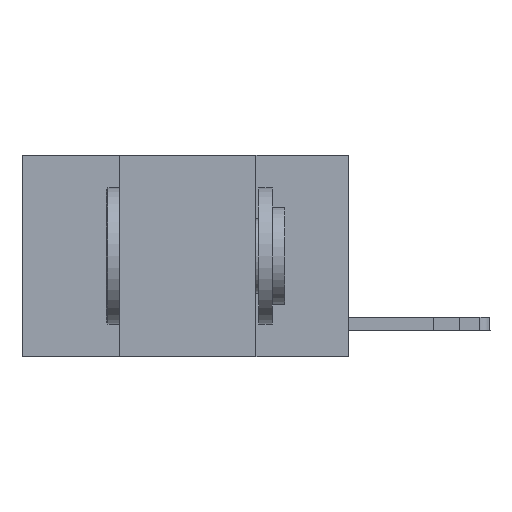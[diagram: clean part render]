
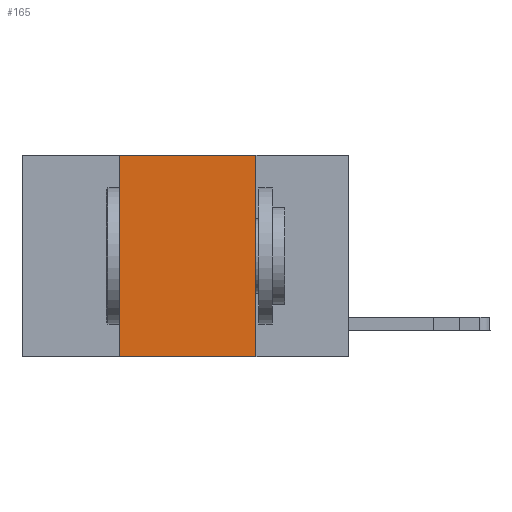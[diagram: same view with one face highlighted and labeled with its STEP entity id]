
A CAD part, left-side view. The second image highlights one B-rep face of the part: STEP entity #165.
In plain terms, the highlighted planar face has unit normal (-1, 0, 0).
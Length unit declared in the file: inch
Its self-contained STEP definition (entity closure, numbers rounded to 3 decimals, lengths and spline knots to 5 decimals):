
#32 = LINE ( 'NONE', #14705, #11902 ) ;
#165 = ADVANCED_FACE ( 'NONE', ( #14296 ), #7506, .F. ) ;
#286 = DIRECTION ( 'NONE',  ( 0., 0., -1. ) ) ;
#1054 = VERTEX_POINT ( 'NONE', #12164 ) ;
#1081 = DIRECTION ( 'NONE',  ( 0., 0., -1. ) ) ;
#1426 = CARTESIAN_POINT ( 'NONE',  ( 0., 0.17, 0. ) ) ;
#1650 = DIRECTION ( 'NONE',  ( 0., 0., 1. ) ) ;
#1777 = EDGE_LOOP ( 'NONE', ( #5308, #9752, #3244, #13307 ) ) ;
#1889 = LINE ( 'NONE', #4613, #5074 ) ;
#1970 = EDGE_CURVE ( 'NONE', #2751, #3465, #32, .T. ) ;
#2751 = VERTEX_POINT ( 'NONE', #1426 ) ;
#3244 = ORIENTED_EDGE ( 'NONE', *, *, #13881, .F. ) ;
#3465 = VERTEX_POINT ( 'NONE', #9005 ) ;
#3810 = CARTESIAN_POINT ( 'NONE',  ( 0., 0.6, 0. ) ) ;
#4613 = CARTESIAN_POINT ( 'NONE',  ( 0., 0.6, -0.37 ) ) ;
#4658 = VECTOR ( 'NONE', #1650, 39.37008 ) ;
#4887 = VECTOR ( 'NONE', #6370, 39.37008 ) ;
#4927 = CARTESIAN_POINT ( 'NONE',  ( 0., 0.6, 0. ) ) ;
#5074 = VECTOR ( 'NONE', #6948, 39.37008 ) ;
#5227 = VERTEX_POINT ( 'NONE', #6787 ) ;
#5308 = ORIENTED_EDGE ( 'NONE', *, *, #1970, .F. ) ;
#6046 = DIRECTION ( 'NONE',  ( 1., 0., 0. ) ) ;
#6195 = LINE ( 'NONE', #3810, #4887 ) ;
#6370 = DIRECTION ( 'NONE',  ( 0., -1., 0. ) ) ;
#6787 = CARTESIAN_POINT ( 'NONE',  ( 0., 0.42, -0.37 ) ) ;
#6948 = DIRECTION ( 'NONE',  ( 0., -1., 0. ) ) ;
#7162 = EDGE_CURVE ( 'NONE', #5227, #3465, #1889, .T. ) ;
#7506 = PLANE ( 'NONE',  #15822 ) ;
#9005 = CARTESIAN_POINT ( 'NONE',  ( 0., 0.17, -0.37 ) ) ;
#9684 = LINE ( 'NONE', #10653, #4658 ) ;
#9752 = ORIENTED_EDGE ( 'NONE', *, *, #10491, .F. ) ;
#10491 = EDGE_CURVE ( 'NONE', #1054, #2751, #6195, .T. ) ;
#10653 = CARTESIAN_POINT ( 'NONE',  ( 0., 0.42, 0. ) ) ;
#11902 = VECTOR ( 'NONE', #286, 39.37008 ) ;
#12164 = CARTESIAN_POINT ( 'NONE',  ( 0., 0.42, 0. ) ) ;
#13307 = ORIENTED_EDGE ( 'NONE', *, *, #7162, .T. ) ;
#13881 = EDGE_CURVE ( 'NONE', #5227, #1054, #9684, .T. ) ;
#14296 = FACE_OUTER_BOUND ( 'NONE', #1777, .T. ) ;
#14705 = CARTESIAN_POINT ( 'NONE',  ( 0., 0.17, 0. ) ) ;
#15822 = AXIS2_PLACEMENT_3D ( 'NONE', #4927, #6046, #1081 ) ;
